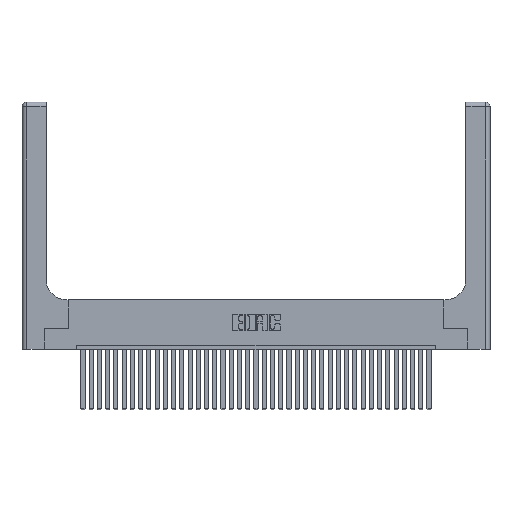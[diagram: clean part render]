
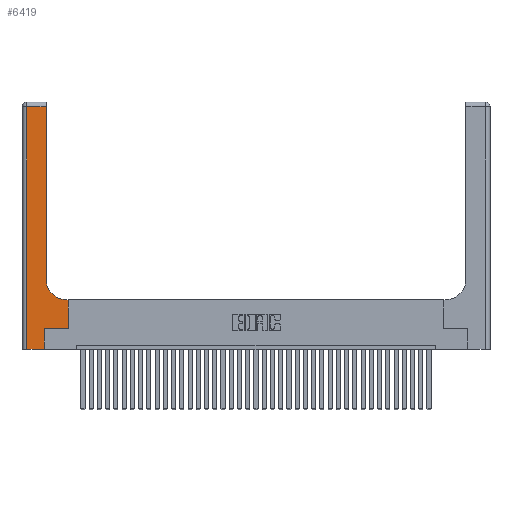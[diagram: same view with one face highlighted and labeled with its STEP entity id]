
A CAD part, top view. The second image highlights one B-rep face of the part: STEP entity #6419.
In plain terms, the highlighted planar face has unit normal (0, 0, 1).
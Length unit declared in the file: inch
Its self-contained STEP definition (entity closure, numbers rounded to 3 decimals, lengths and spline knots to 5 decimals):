
#451 = CARTESIAN_POINT ( 'NONE',  ( 0., 2.94, 0.37 ) ) ;
#859 = VERTEX_POINT ( 'NONE', #11341 ) ;
#1475 = VERTEX_POINT ( 'NONE', #6580 ) ;
#1994 = EDGE_CURVE ( 'NONE', #15527, #3593, #16307, .T. ) ;
#2309 = DIRECTION ( 'NONE',  ( 0., 1., 0. ) ) ;
#2576 = VERTEX_POINT ( 'NONE', #10076 ) ;
#3593 = VERTEX_POINT ( 'NONE', #5966 ) ;
#3741 = AXIS2_PLACEMENT_3D ( 'NONE', #24847, #27716, #13444 ) ;
#3962 = ORIENTED_EDGE ( 'NONE', *, *, #19021, .T. ) ;
#4149 = CARTESIAN_POINT ( 'NONE',  ( 0.2915, 3., 0.37 ) ) ;
#4614 = DIRECTION ( 'NONE',  ( 0., -1., 0. ) ) ;
#5078 = VECTOR ( 'NONE', #34660, 39.37008 ) ;
#5295 = LINE ( 'NONE', #451, #32195 ) ;
#5492 = VECTOR ( 'NONE', #12225, 39.37008 ) ;
#5768 = CARTESIAN_POINT ( 'NONE',  ( 0.06, 0., 0.37 ) ) ;
#5966 = CARTESIAN_POINT ( 'NONE',  ( 0.269, 0.25, 0.37 ) ) ;
#6041 = LINE ( 'NONE', #4149, #31654 ) ;
#6253 = ORIENTED_EDGE ( 'NONE', *, *, #1994, .T. ) ;
#6419 = ADVANCED_FACE ( 'NONE', ( #18489 ), #22448, .F. ) ;
#6580 = CARTESIAN_POINT ( 'NONE',  ( 0.2915, 2.94, 0.37 ) ) ;
#6892 = DIRECTION ( 'NONE',  ( -1., 0., 0. ) ) ;
#7746 = VERTEX_POINT ( 'NONE', #18035 ) ;
#8221 = LINE ( 'NONE', #28616, #5078 ) ;
#9607 = CARTESIAN_POINT ( 'NONE',  ( 0.269, 0.25, 0.37 ) ) ;
#9813 = VECTOR ( 'NONE', #23974, 39.37008 ) ;
#10059 = DIRECTION ( 'NONE',  ( 0., 1., 0. ) ) ;
#10076 = CARTESIAN_POINT ( 'NONE',  ( 0.2915, 0.85, 0.37 ) ) ;
#10137 = CARTESIAN_POINT ( 'NONE',  ( 0.06, 3., 0.37 ) ) ;
#10972 = VERTEX_POINT ( 'NONE', #5768 ) ;
#11111 = VECTOR ( 'NONE', #6892, 39.37008 ) ;
#11341 = CARTESIAN_POINT ( 'NONE',  ( 0.5585, 0.6, 0.37 ) ) ;
#12225 = DIRECTION ( 'NONE',  ( 1., 0., 0. ) ) ;
#12937 = DIRECTION ( 'NONE',  ( 0., 0., -1. ) ) ;
#13444 = DIRECTION ( 'NONE',  ( -1., 0., 0. ) ) ;
#13619 = VECTOR ( 'NONE', #2309, 39.37008 ) ;
#13695 = EDGE_CURVE ( 'NONE', #7746, #2576, #30458, .T. ) ;
#14549 = DIRECTION ( 'NONE',  ( -1., 0., 0. ) ) ;
#15527 = VERTEX_POINT ( 'NONE', #35082 ) ;
#15571 = VERTEX_POINT ( 'NONE', #18155 ) ;
#16185 = ORIENTED_EDGE ( 'NONE', *, *, #24723, .T. ) ;
#16287 = VECTOR ( 'NONE', #4614, 39.37008 ) ;
#16307 = LINE ( 'NONE', #31164, #13619 ) ;
#18035 = CARTESIAN_POINT ( 'NONE',  ( 0.5415, 0.6, 0.37 ) ) ;
#18087 = CARTESIAN_POINT ( 'NONE',  ( 0., 0., 0.37 ) ) ;
#18155 = CARTESIAN_POINT ( 'NONE',  ( 0.06, 2.94, 0.37 ) ) ;
#18198 = ORIENTED_EDGE ( 'NONE', *, *, #29301, .T. ) ;
#18489 = FACE_OUTER_BOUND ( 'NONE', #19874, .T. ) ;
#18515 = LINE ( 'NONE', #10137, #16287 ) ;
#19012 = EDGE_CURVE ( 'NONE', #1475, #15571, #5295, .T. ) ;
#19021 = EDGE_CURVE ( 'NONE', #859, #7746, #29958, .T. ) ;
#19653 = ORIENTED_EDGE ( 'NONE', *, *, #13695, .T. ) ;
#19874 = EDGE_LOOP ( 'NONE', ( #18198, #26944, #28472, #33477, #6253, #24823, #16185, #3962, #19653 ) ) ;
#21451 = CARTESIAN_POINT ( 'NONE',  ( 0.5415, 0.85, 0.37 ) ) ;
#21674 = LINE ( 'NONE', #9607, #5492 ) ;
#22448 = PLANE ( 'NONE',  #3741 ) ;
#23735 = LINE ( 'NONE', #18087, #9813 ) ;
#23974 = DIRECTION ( 'NONE',  ( 1., 0., 0. ) ) ;
#24569 = EDGE_CURVE ( 'NONE', #3593, #25132, #21674, .T. ) ;
#24723 = EDGE_CURVE ( 'NONE', #25132, #859, #8221, .T. ) ;
#24823 = ORIENTED_EDGE ( 'NONE', *, *, #24569, .T. ) ;
#24847 = CARTESIAN_POINT ( 'NONE',  ( 0., 3., 0.37 ) ) ;
#25132 = VERTEX_POINT ( 'NONE', #36023 ) ;
#25860 = AXIS2_PLACEMENT_3D ( 'NONE', #21451, #12937, #27475 ) ;
#26439 = EDGE_CURVE ( 'NONE', #10972, #15527, #23735, .T. ) ;
#26944 = ORIENTED_EDGE ( 'NONE', *, *, #19012, .T. ) ;
#27475 = DIRECTION ( 'NONE',  ( 1., 0., 0. ) ) ;
#27716 = DIRECTION ( 'NONE',  ( 0., 0., -1. ) ) ;
#28472 = ORIENTED_EDGE ( 'NONE', *, *, #31280, .T. ) ;
#28594 = CARTESIAN_POINT ( 'NONE',  ( 0.2915, 0.6, 0.37 ) ) ;
#28616 = CARTESIAN_POINT ( 'NONE',  ( 0.5585, 0.25, 0.37 ) ) ;
#29301 = EDGE_CURVE ( 'NONE', #2576, #1475, #6041, .T. ) ;
#29958 = LINE ( 'NONE', #28594, #11111 ) ;
#30458 = CIRCLE ( 'NONE', #25860, 0.25 ) ;
#31164 = CARTESIAN_POINT ( 'NONE',  ( 0.269, 0., 0.37 ) ) ;
#31280 = EDGE_CURVE ( 'NONE', #15571, #10972, #18515, .T. ) ;
#31654 = VECTOR ( 'NONE', #10059, 39.37008 ) ;
#32195 = VECTOR ( 'NONE', #14549, 39.37008 ) ;
#33477 = ORIENTED_EDGE ( 'NONE', *, *, #26439, .T. ) ;
#34660 = DIRECTION ( 'NONE',  ( 0., 1., 0. ) ) ;
#35082 = CARTESIAN_POINT ( 'NONE',  ( 0.269, 0., 0.37 ) ) ;
#36023 = CARTESIAN_POINT ( 'NONE',  ( 0.5585, 0.25, 0.37 ) ) ;
